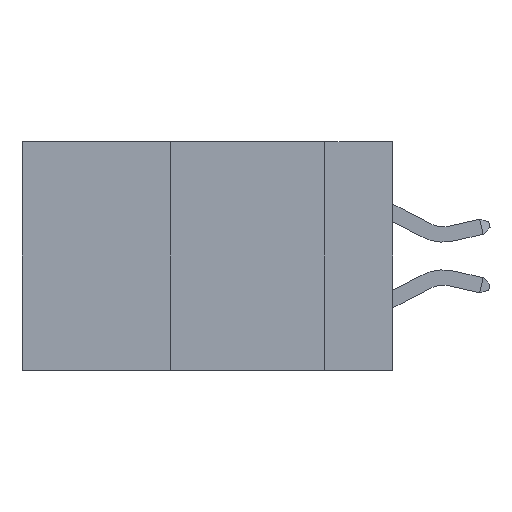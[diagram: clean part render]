
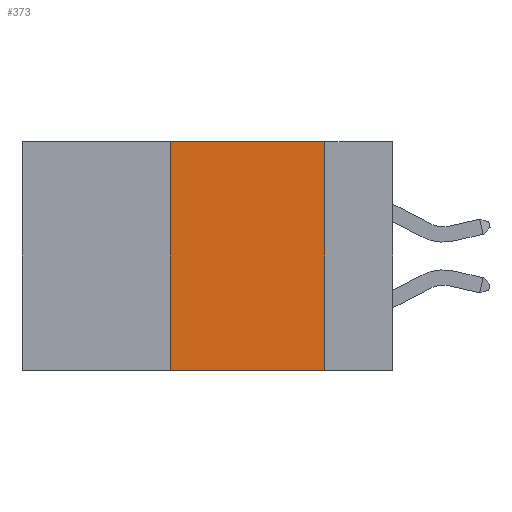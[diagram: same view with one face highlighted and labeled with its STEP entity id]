
A CAD part, left-side view. The second image highlights one B-rep face of the part: STEP entity #373.
In plain terms, the highlighted planar face has unit normal (-1, 0, 0).
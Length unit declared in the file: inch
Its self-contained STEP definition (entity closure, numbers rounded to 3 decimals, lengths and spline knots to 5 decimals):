
#55 = CARTESIAN_POINT ( 'NONE',  ( 0., 0.36, -0.37 ) ) ;
#373 = ADVANCED_FACE ( 'NONE', ( #2117 ), #1413, .F. ) ;
#1003 = VERTEX_POINT ( 'NONE', #8267 ) ;
#1143 = VECTOR ( 'NONE', #5786, 39.37008 ) ;
#1413 = PLANE ( 'NONE',  #8775 ) ;
#1553 = VECTOR ( 'NONE', #8453, 39.37008 ) ;
#1821 = ORIENTED_EDGE ( 'NONE', *, *, #3580, .F. ) ;
#2101 = DIRECTION ( 'NONE',  ( 0., -1., 0. ) ) ;
#2117 = FACE_OUTER_BOUND ( 'NONE', #11383, .T. ) ;
#2950 = CARTESIAN_POINT ( 'NONE',  ( 0., 0.11, 0. ) ) ;
#3171 = LINE ( 'NONE', #3694, #10408 ) ;
#3328 = EDGE_CURVE ( 'NONE', #8770, #7420, #7331, .T. ) ;
#3347 = EDGE_CURVE ( 'NONE', #11119, #7420, #6746, .T. ) ;
#3413 = ORIENTED_EDGE ( 'NONE', *, *, #3347, .F. ) ;
#3580 = EDGE_CURVE ( 'NONE', #8770, #1003, #3171, .T. ) ;
#3662 = CARTESIAN_POINT ( 'NONE',  ( 0., 0.6, -0.37 ) ) ;
#3694 = CARTESIAN_POINT ( 'NONE',  ( 0., 0.36, 0. ) ) ;
#3888 = ORIENTED_EDGE ( 'NONE', *, *, #3328, .T. ) ;
#4746 = ORIENTED_EDGE ( 'NONE', *, *, #5503, .F. ) ;
#5194 = LINE ( 'NONE', #12285, #1143 ) ;
#5503 = EDGE_CURVE ( 'NONE', #1003, #11119, #5194, .T. ) ;
#5786 = DIRECTION ( 'NONE',  ( 0., -1., 0. ) ) ;
#5993 = CARTESIAN_POINT ( 'NONE',  ( 0., 0.11, 0. ) ) ;
#6746 = LINE ( 'NONE', #5993, #1553 ) ;
#7331 = LINE ( 'NONE', #3662, #11953 ) ;
#7420 = VERTEX_POINT ( 'NONE', #10797 ) ;
#8267 = CARTESIAN_POINT ( 'NONE',  ( 0., 0.36, 0. ) ) ;
#8325 = CARTESIAN_POINT ( 'NONE',  ( 0., 0.6, 0. ) ) ;
#8453 = DIRECTION ( 'NONE',  ( 0., 0., -1. ) ) ;
#8770 = VERTEX_POINT ( 'NONE', #55 ) ;
#8775 = AXIS2_PLACEMENT_3D ( 'NONE', #8325, #9179, #9419 ) ;
#9179 = DIRECTION ( 'NONE',  ( 1., 0., 0. ) ) ;
#9419 = DIRECTION ( 'NONE',  ( 0., 0., -1. ) ) ;
#10408 = VECTOR ( 'NONE', #10409, 39.37008 ) ;
#10409 = DIRECTION ( 'NONE',  ( 0., 0., 1. ) ) ;
#10797 = CARTESIAN_POINT ( 'NONE',  ( 0., 0.11, -0.37 ) ) ;
#11119 = VERTEX_POINT ( 'NONE', #2950 ) ;
#11383 = EDGE_LOOP ( 'NONE', ( #3413, #4746, #1821, #3888 ) ) ;
#11953 = VECTOR ( 'NONE', #2101, 39.37008 ) ;
#12285 = CARTESIAN_POINT ( 'NONE',  ( 0., 0.6, 0. ) ) ;
